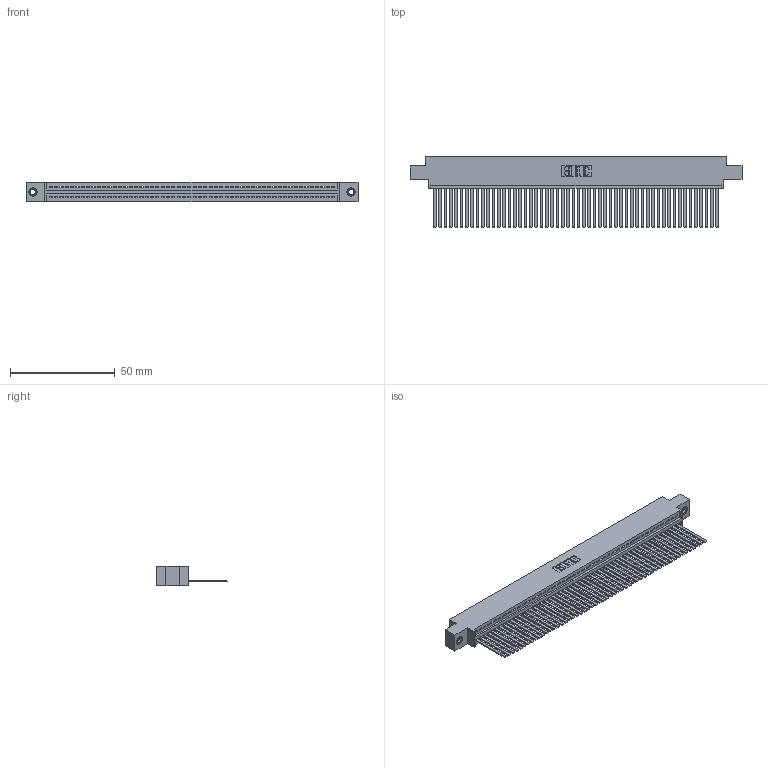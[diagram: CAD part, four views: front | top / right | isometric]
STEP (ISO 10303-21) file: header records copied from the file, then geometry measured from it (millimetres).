
FILE_DESCRIPTION (( 'STEP AP203' ), '1' );
FILE_NAME ('395-054-544-607.STEP', '2018-11-21T10:59:51', ( '' ), ( '' ), 'SwSTEP 2.0', 'SolidWorks 2016', '' );
FILE_SCHEMA (( 'CONFIG_CONTROL_DESIGN' ));
Length unit declared in the file: inch
Products named in the file (4): 345 Part_0.170 Offset - 0.156 Dia-TI; 345-250-001_345-250-005-103; 395-054-544-607; 345-292-001_345-293-144
Assembly tree (57 placements, depth 2):
  395-054-544-607
    345 Part_0.170 Offset - 0.156 Dia-TI
    345-292-001_345-293-144  x54
    345-250-001_345-250-005-103  x2
Bounding box: 158.37 x 33.96 x 9.4 mm (x, y, z)
Volume: 15638.8 mm3; surface area: 22982.3 mm2
Topology: 57 solids, 57 shells, 2998 faces, 9021 edges, 5934 vertices
Faces by surface type: plane 2060, cylinder 922, cone 12, torus 4
Entity records: 40160 total; most frequent: CARTESIAN_POINT 6937, ORIENTED_EDGE 6918, DIRECTION 6065, EDGE_CURVE 3459, VECTOR 3095, LINE 3095, VERTEX_POINT 2300, AXIS2_PLACEMENT_3D 1485
